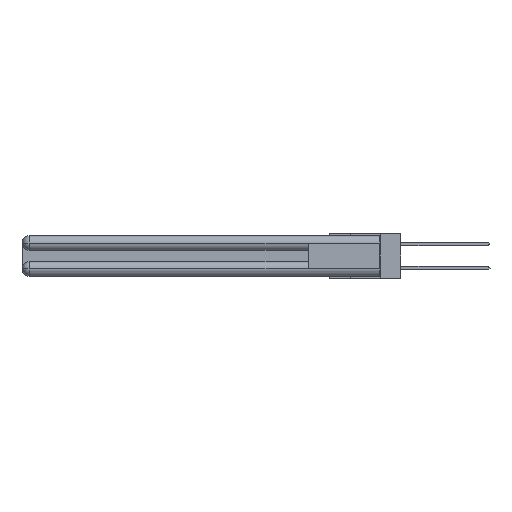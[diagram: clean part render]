
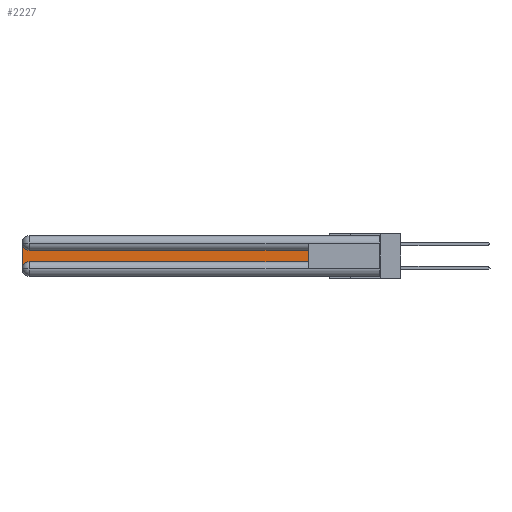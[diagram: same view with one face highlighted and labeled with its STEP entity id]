
A CAD part, left-side view. The second image highlights one B-rep face of the part: STEP entity #2227.
In plain terms, the highlighted planar face has unit normal (-1, 0, 0).
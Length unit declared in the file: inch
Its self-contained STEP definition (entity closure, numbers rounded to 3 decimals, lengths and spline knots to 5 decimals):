
#572 = EDGE_CURVE ( 'NONE', #5587, #5517, #7677, .T. ) ;
#1050 = DIRECTION ( 'NONE',  ( 0., 0., -1. ) ) ;
#1058 = ORIENTED_EDGE ( 'NONE', *, *, #572, .T. ) ;
#1247 = CIRCLE ( 'NONE', #29768, 0.06 ) ;
#2143 = CARTESIAN_POINT ( 'NONE',  ( 0.075, 0.6, -0.2175 ) ) ;
#2203 = EDGE_CURVE ( 'NONE', #28385, #2420, #8384, .T. ) ;
#2227 = ADVANCED_FACE ( 'NONE', ( #23763 ), #8241, .F. ) ;
#2420 = VERTEX_POINT ( 'NONE', #14830 ) ;
#3285 = AXIS2_PLACEMENT_3D ( 'NONE', #4555, #24821, #14705 ) ;
#3599 = CARTESIAN_POINT ( 'NONE',  ( 0.075, 3., -0.2175 ) ) ;
#4555 = CARTESIAN_POINT ( 'NONE',  ( 0.075, 2.94, -0.0625 ) ) ;
#4561 = EDGE_LOOP ( 'NONE', ( #5784, #31028, #15481, #12927, #6078, #1058 ) ) ;
#5517 = VERTEX_POINT ( 'NONE', #24981 ) ;
#5587 = VERTEX_POINT ( 'NONE', #8362 ) ;
#5784 = ORIENTED_EDGE ( 'NONE', *, *, #12255, .T. ) ;
#6078 = ORIENTED_EDGE ( 'NONE', *, *, #8311, .T. ) ;
#6336 = DIRECTION ( 'NONE',  ( 1., 0., 0. ) ) ;
#7677 = LINE ( 'NONE', #12398, #22256 ) ;
#7963 = VECTOR ( 'NONE', #1050, 39.37008 ) ;
#8241 = PLANE ( 'NONE',  #27184 ) ;
#8311 = EDGE_CURVE ( 'NONE', #10666, #5587, #15595, .T. ) ;
#8362 = CARTESIAN_POINT ( 'NONE',  ( 0.075, 0.6, -0.2175 ) ) ;
#8384 = LINE ( 'NONE', #3599, #7963 ) ;
#9023 = EDGE_CURVE ( 'NONE', #26132, #28385, #9578, .T. ) ;
#9514 = DIRECTION ( 'NONE',  ( 0., 0., 1. ) ) ;
#9578 = CIRCLE ( 'NONE', #3285, 0.06 ) ;
#10666 = VERTEX_POINT ( 'NONE', #31249 ) ;
#12255 = EDGE_CURVE ( 'NONE', #5517, #26132, #30835, .T. ) ;
#12398 = CARTESIAN_POINT ( 'NONE',  ( 0.075, 0.6, -0.2175 ) ) ;
#12927 = ORIENTED_EDGE ( 'NONE', *, *, #30038, .T. ) ;
#14705 = DIRECTION ( 'NONE',  ( 0., 0., -1. ) ) ;
#14830 = CARTESIAN_POINT ( 'NONE',  ( 0.075, 3., -0.2775 ) ) ;
#15333 = CARTESIAN_POINT ( 'NONE',  ( 0.075, 0.6, -0.1225 ) ) ;
#15481 = ORIENTED_EDGE ( 'NONE', *, *, #2203, .T. ) ;
#15595 = LINE ( 'NONE', #2143, #30117 ) ;
#16503 = CARTESIAN_POINT ( 'NONE',  ( 0.075, 3., -0.1225 ) ) ;
#17885 = VECTOR ( 'NONE', #20309, 39.37008 ) ;
#19154 = DIRECTION ( 'NONE',  ( 1., 0., 0. ) ) ;
#20309 = DIRECTION ( 'NONE',  ( 0., 1., 0. ) ) ;
#22256 = VECTOR ( 'NONE', #9514, 39.37008 ) ;
#22387 = CARTESIAN_POINT ( 'NONE',  ( 0.075, 2.94, -0.1225 ) ) ;
#22547 = DIRECTION ( 'NONE',  ( 0., -1., 0. ) ) ;
#23640 = CARTESIAN_POINT ( 'NONE',  ( 0.075, 3., -0.0625 ) ) ;
#23763 = FACE_OUTER_BOUND ( 'NONE', #4561, .T. ) ;
#24821 = DIRECTION ( 'NONE',  ( 1., 0., 0. ) ) ;
#24981 = CARTESIAN_POINT ( 'NONE',  ( 0.075, 0.6, -0.1225 ) ) ;
#26132 = VERTEX_POINT ( 'NONE', #22387 ) ;
#27184 = AXIS2_PLACEMENT_3D ( 'NONE', #16503, #6336, #28771 ) ;
#28385 = VERTEX_POINT ( 'NONE', #23640 ) ;
#28771 = DIRECTION ( 'NONE',  ( 0., 0., -1. ) ) ;
#28890 = CARTESIAN_POINT ( 'NONE',  ( 0.075, 2.94, -0.2775 ) ) ;
#29003 = DIRECTION ( 'NONE',  ( 0., 0., -1. ) ) ;
#29768 = AXIS2_PLACEMENT_3D ( 'NONE', #28890, #19154, #29003 ) ;
#30038 = EDGE_CURVE ( 'NONE', #2420, #10666, #1247, .T. ) ;
#30117 = VECTOR ( 'NONE', #22547, 39.37008 ) ;
#30835 = LINE ( 'NONE', #15333, #17885 ) ;
#31028 = ORIENTED_EDGE ( 'NONE', *, *, #9023, .T. ) ;
#31249 = CARTESIAN_POINT ( 'NONE',  ( 0.075, 2.94, -0.2175 ) ) ;
